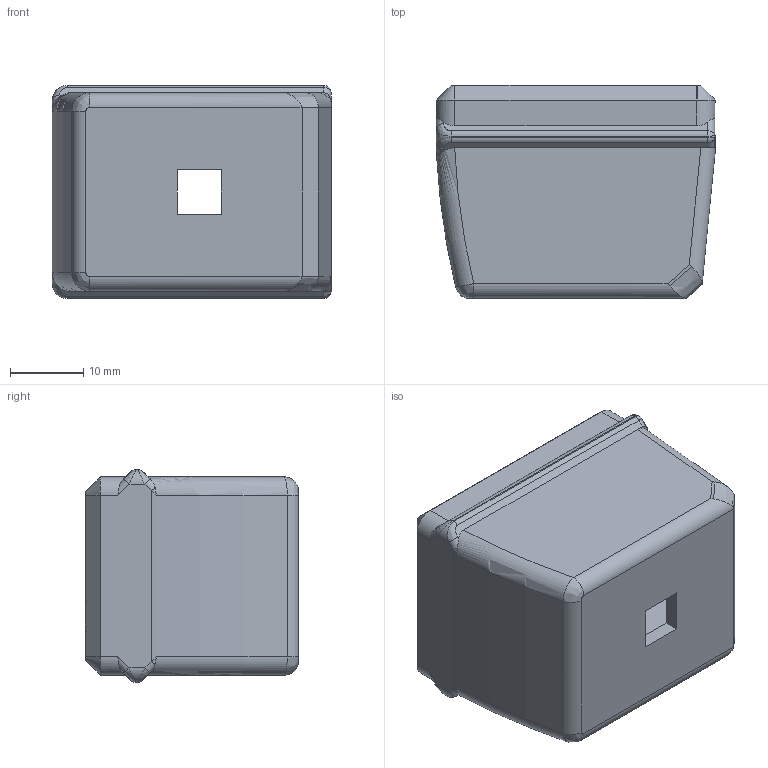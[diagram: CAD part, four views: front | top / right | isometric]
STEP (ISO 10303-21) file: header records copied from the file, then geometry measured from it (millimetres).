
FILE_DESCRIPTION(/* description */ (''),/* implementation_level */ '2;1');
FILE_NAME(/* name */ 'vz61 +5 Mag Extension.step',/* time_stamp */ '2021-02-09T08:48:10-07:00',/* author */ (''),/* organization */ (''),/* preprocessor_version */ 'ST-DEVELOPER v18.1',/* originating_system */ 'Autodesk Translation Framework v9.7.1.1290',/* authorisation */ '');
FILE_SCHEMA (('AUTOMOTIVE_DESIGN { 1 0 10303 214 3 1 1 }'));
Length unit declared in the file: millimetre
Products named in the file (1): vz61 Mag Extension 5
Bounding box: 38 x 29 x 29 mm (x, y, z)
Volume: 12396.7 mm3; surface area: 8076.2 mm2
Topology: 1 solids, 1 shells, 103 faces, 263 edges, 162 vertices
Faces by surface type: plane 42, cylinder 25, bspline 20, torus 10, sphere 4, cone 2
Entity records: 4216 total; most frequent: CARTESIAN_POINT 1798, ORIENTED_EDGE 526, DIRECTION 457, EDGE_CURVE 263, AXIS2_PLACEMENT_3D 163, VERTEX_POINT 162, LINE 131, VECTOR 131
